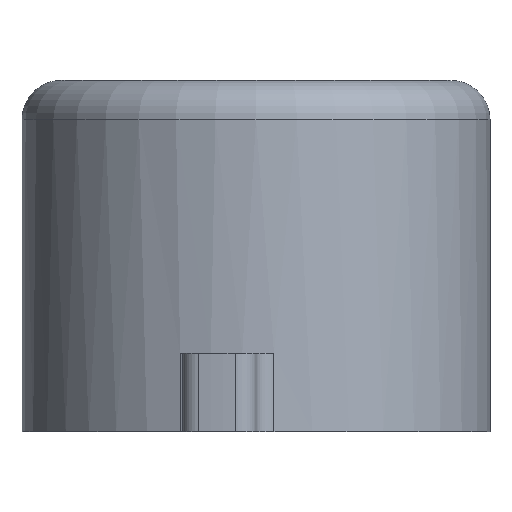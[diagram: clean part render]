
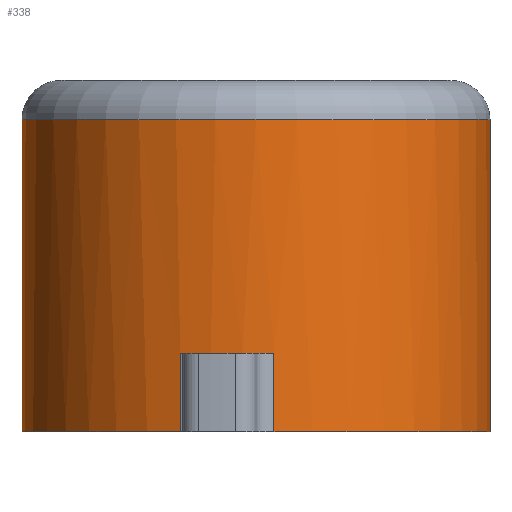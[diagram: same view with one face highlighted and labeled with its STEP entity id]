
A CAD part, front view. The second image highlights one B-rep face of the part: STEP entity #338.
In plain terms, the highlighted cylindrical face has radius 22.5 mm (diameter 45 mm), a partial arc.
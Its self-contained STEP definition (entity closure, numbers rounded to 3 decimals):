
#20 = ORIENTED_EDGE ( 'NONE', *, *, #448, .T. ) ;
#42 = DIRECTION ( 'NONE',  ( 0., 0., -1. ) ) ;
#45 = CARTESIAN_POINT ( 'NONE',  ( 0., 0., 5.532 ) ) ;
#50 = ORIENTED_EDGE ( 'NONE', *, *, #762, .T. ) ;
#51 = CIRCLE ( 'NONE', #916, 22.5 ) ;
#77 = DIRECTION ( 'NONE',  ( 1., 0., 0. ) ) ;
#78 = VECTOR ( 'NONE', #1005, 1000. ) ;
#89 = LINE ( 'NONE', #1019, #78 ) ;
#91 = DIRECTION ( 'NONE',  ( 0., 0., -1. ) ) ;
#96 = CARTESIAN_POINT ( 'NONE',  ( 0., 0., 39.282 ) ) ;
#97 = DIRECTION ( 'NONE',  ( -1., 0., 0. ) ) ;
#98 = CARTESIAN_POINT ( 'NONE',  ( -22.5, 0., 5.532 ) ) ;
#108 = DIRECTION ( 'NONE',  ( 0., 0., -1. ) ) ;
#109 = DIRECTION ( 'NONE',  ( 0., 0., 1. ) ) ;
#112 = CARTESIAN_POINT ( 'NONE',  ( -22.5, 0., 39.282 ) ) ;
#122 = DIRECTION ( 'NONE',  ( 1., 0., 0. ) ) ;
#123 = CARTESIAN_POINT ( 'NONE',  ( 0., 0., 5.532 ) ) ;
#148 = VERTEX_POINT ( 'NONE', #753 ) ;
#196 = DIRECTION ( 'NONE',  ( 0., 0., 1. ) ) ;
#205 = CYLINDRICAL_SURFACE ( 'NONE', #398, 22.5 ) ;
#224 = DIRECTION ( 'NONE',  ( 0., 0., -1. ) ) ;
#228 = ORIENTED_EDGE ( 'NONE', *, *, #882, .F. ) ;
#236 = FACE_OUTER_BOUND ( 'NONE', #697, .T. ) ;
#247 = CARTESIAN_POINT ( 'NONE',  ( 22.5, 0., 39.282 ) ) ;
#273 = VERTEX_POINT ( 'NONE', #312 ) ;
#277 = EDGE_CURVE ( 'NONE', #148, #377, #385, .T. ) ;
#282 = VECTOR ( 'NONE', #108, 1000. ) ;
#307 = DIRECTION ( 'NONE',  ( 0., 0., -1. ) ) ;
#311 = CARTESIAN_POINT ( 'NONE',  ( 1.731, -22.433, 13.032 ) ) ;
#312 = CARTESIAN_POINT ( 'NONE',  ( -7.292, -21.285, 13.032 ) ) ;
#328 = EDGE_CURVE ( 'NONE', #940, #847, #404, .T. ) ;
#338 = ADVANCED_FACE ( 'NONE', ( #236 ), #205, .T. ) ;
#347 = VECTOR ( 'NONE', #224, 1000. ) ;
#359 = AXIS2_PLACEMENT_3D ( 'NONE', #45, #960, #122 ) ;
#377 = VERTEX_POINT ( 'NONE', #1052 ) ;
#385 = LINE ( 'NONE', #247, #347 ) ;
#398 = AXIS2_PLACEMENT_3D ( 'NONE', #96, #91, #97 ) ;
#404 = LINE ( 'NONE', #112, #282 ) ;
#429 = AXIS2_PLACEMENT_3D ( 'NONE', #123, #109, #77 ) ;
#448 = EDGE_CURVE ( 'NONE', #1018, #919, #89, .T. ) ;
#461 = CIRCLE ( 'NONE', #577, 22.5 ) ;
#568 = DIRECTION ( 'NONE',  ( 1., 0., 0. ) ) ;
#577 = AXIS2_PLACEMENT_3D ( 'NONE', #879, #42, #568 ) ;
#588 = CARTESIAN_POINT ( 'NONE',  ( -22.5, 0., 35.532 ) ) ;
#595 = CIRCLE ( 'NONE', #359, 22.5 ) ;
#646 = EDGE_CURVE ( 'NONE', #847, #804, #1043, .T. ) ;
#672 = CARTESIAN_POINT ( 'NONE',  ( -7.292, -21.285, 5.532 ) ) ;
#685 = VECTOR ( 'NONE', #196, 1000. ) ;
#697 = EDGE_LOOP ( 'NONE', ( #1020, #50, #797, #867, #1081, #228, #20, #758 ) ) ;
#721 = CARTESIAN_POINT ( 'NONE',  ( 0., 0., 13.032 ) ) ;
#738 = CARTESIAN_POINT ( 'NONE',  ( -7.292, -21.285, 39.282 ) ) ;
#753 = CARTESIAN_POINT ( 'NONE',  ( 22.5, 0., 35.532 ) ) ;
#758 = ORIENTED_EDGE ( 'NONE', *, *, #850, .T. ) ;
#762 = EDGE_CURVE ( 'NONE', #148, #940, #461, .T. ) ;
#790 = LINE ( 'NONE', #738, #685 ) ;
#797 = ORIENTED_EDGE ( 'NONE', *, *, #328, .T. ) ;
#804 = VERTEX_POINT ( 'NONE', #672 ) ;
#811 = DIRECTION ( 'NONE',  ( -1., 0., 0. ) ) ;
#847 = VERTEX_POINT ( 'NONE', #98 ) ;
#850 = EDGE_CURVE ( 'NONE', #919, #377, #595, .T. ) ;
#867 = ORIENTED_EDGE ( 'NONE', *, *, #646, .T. ) ;
#879 = CARTESIAN_POINT ( 'NONE',  ( 0., 0., 35.532 ) ) ;
#882 = EDGE_CURVE ( 'NONE', #1018, #273, #51, .T. ) ;
#896 = CARTESIAN_POINT ( 'NONE',  ( 1.731, -22.433, 5.532 ) ) ;
#916 = AXIS2_PLACEMENT_3D ( 'NONE', #721, #307, #811 ) ;
#919 = VERTEX_POINT ( 'NONE', #896 ) ;
#940 = VERTEX_POINT ( 'NONE', #588 ) ;
#960 = DIRECTION ( 'NONE',  ( 0., 0., 1. ) ) ;
#978 = EDGE_CURVE ( 'NONE', #804, #273, #790, .T. ) ;
#1005 = DIRECTION ( 'NONE',  ( 0., 0., -1. ) ) ;
#1018 = VERTEX_POINT ( 'NONE', #311 ) ;
#1019 = CARTESIAN_POINT ( 'NONE',  ( 1.731, -22.433, 39.282 ) ) ;
#1020 = ORIENTED_EDGE ( 'NONE', *, *, #277, .F. ) ;
#1043 = CIRCLE ( 'NONE', #429, 22.5 ) ;
#1052 = CARTESIAN_POINT ( 'NONE',  ( 22.5, 0., 5.532 ) ) ;
#1081 = ORIENTED_EDGE ( 'NONE', *, *, #978, .T. ) ;
